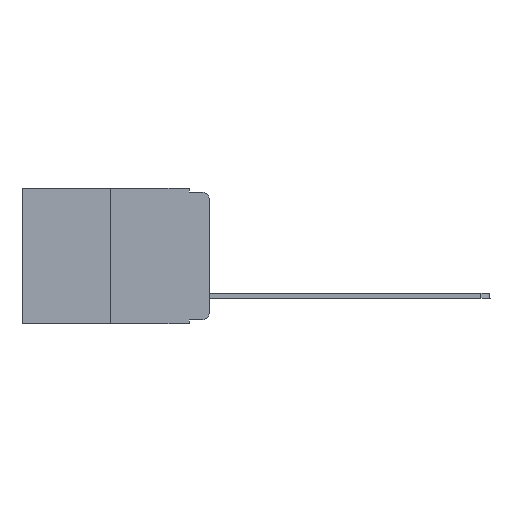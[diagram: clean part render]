
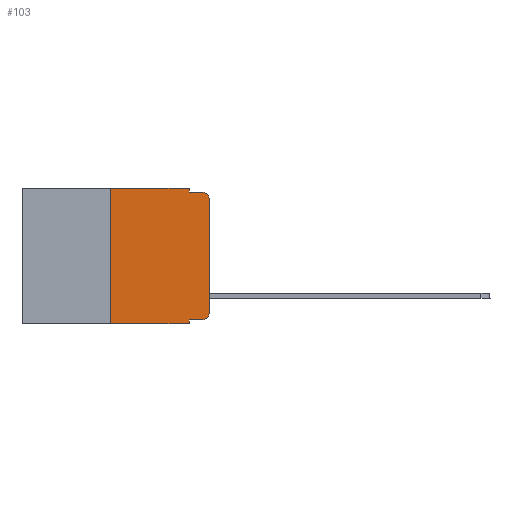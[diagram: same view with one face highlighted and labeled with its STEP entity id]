
A CAD part, left-side view. The second image highlights one B-rep face of the part: STEP entity #103.
In plain terms, the highlighted planar face has unit normal (-1, 0, 0).
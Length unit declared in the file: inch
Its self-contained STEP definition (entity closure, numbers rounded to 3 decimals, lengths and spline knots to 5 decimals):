
#103 = ADVANCED_FACE ( 'NONE', ( #1729 ), #5433, .F. ) ;
#255 = CARTESIAN_POINT ( 'NONE',  ( 0., 0.051, 0. ) ) ;
#349 = CARTESIAN_POINT ( 'NONE',  ( 0., 0.02, -0.01 ) ) ;
#372 = DIRECTION ( 'NONE',  ( 0., 0., -1. ) ) ;
#396 = EDGE_CURVE ( 'NONE', #9102, #11403, #11046, .T. ) ;
#426 = DIRECTION ( 'NONE',  ( 0., -1., 0. ) ) ;
#497 = EDGE_LOOP ( 'NONE', ( #7751, #4472, #10435, #3628, #12451, #8304, #6946, #598, #6780, #918 ) ) ;
#598 = ORIENTED_EDGE ( 'NONE', *, *, #800, .F. ) ;
#708 = VERTEX_POINT ( 'NONE', #5672 ) ;
#800 = EDGE_CURVE ( 'NONE', #7543, #8724, #7452, .T. ) ;
#918 = ORIENTED_EDGE ( 'NONE', *, *, #6258, .T. ) ;
#961 = CARTESIAN_POINT ( 'NONE',  ( 0., 0.051, 0. ) ) ;
#1445 = AXIS2_PLACEMENT_3D ( 'NONE', #3823, #12414, #6648 ) ;
#1504 = VERTEX_POINT ( 'NONE', #4629 ) ;
#1692 = VECTOR ( 'NONE', #6215, 39.37008 ) ;
#1729 = FACE_OUTER_BOUND ( 'NONE', #497, .T. ) ;
#2142 = CARTESIAN_POINT ( 'NONE',  ( 0., 0.051, 0. ) ) ;
#2344 = VECTOR ( 'NONE', #4037, 39.37008 ) ;
#2550 = CARTESIAN_POINT ( 'NONE',  ( 0., 0.02, -0.333 ) ) ;
#2570 = LINE ( 'NONE', #12297, #5564 ) ;
#2687 = EDGE_CURVE ( 'NONE', #11403, #7449, #8014, .T. ) ;
#2717 = DIRECTION ( 'NONE',  ( 1., 0., 0. ) ) ;
#2796 = VECTOR ( 'NONE', #2959, 39.37008 ) ;
#2822 = EDGE_CURVE ( 'NONE', #1504, #8724, #6805, .T. ) ;
#2959 = DIRECTION ( 'NONE',  ( 0., 0., -1. ) ) ;
#3353 = DIRECTION ( 'NONE',  ( 0., -1., 0. ) ) ;
#3569 = LINE ( 'NONE', #10056, #10960 ) ;
#3628 = ORIENTED_EDGE ( 'NONE', *, *, #396, .F. ) ;
#3698 = DIRECTION ( 'NONE',  ( 0., -1., 0. ) ) ;
#3823 = CARTESIAN_POINT ( 'NONE',  ( 0., 0.02, -0.03 ) ) ;
#4037 = DIRECTION ( 'NONE',  ( 0., 0., -1. ) ) ;
#4445 = CARTESIAN_POINT ( 'NONE',  ( 0., 0.051, -0.333 ) ) ;
#4455 = CARTESIAN_POINT ( 'NONE',  ( 0., 0.25, 0. ) ) ;
#4472 = ORIENTED_EDGE ( 'NONE', *, *, #6532, .T. ) ;
#4629 = CARTESIAN_POINT ( 'NONE',  ( 0., 0.25, -0.343 ) ) ;
#5057 = EDGE_CURVE ( 'NONE', #7543, #6416, #3569, .T. ) ;
#5117 = VERTEX_POINT ( 'NONE', #11272 ) ;
#5433 = PLANE ( 'NONE',  #8969 ) ;
#5476 = DIRECTION ( 'NONE',  ( 0., 0., -1. ) ) ;
#5564 = VECTOR ( 'NONE', #9657, 39.37008 ) ;
#5672 = CARTESIAN_POINT ( 'NONE',  ( 0., 0., -0.313 ) ) ;
#6215 = DIRECTION ( 'NONE',  ( 0., -1., 0. ) ) ;
#6258 = EDGE_CURVE ( 'NONE', #6416, #708, #7625, .T. ) ;
#6416 = VERTEX_POINT ( 'NONE', #2550 ) ;
#6532 = EDGE_CURVE ( 'NONE', #5117, #7449, #12420, .T. ) ;
#6605 = EDGE_CURVE ( 'NONE', #708, #5117, #11222, .T. ) ;
#6648 = DIRECTION ( 'NONE',  ( 0., 0., -1. ) ) ;
#6780 = ORIENTED_EDGE ( 'NONE', *, *, #5057, .T. ) ;
#6805 = LINE ( 'NONE', #10054, #1692 ) ;
#6946 = ORIENTED_EDGE ( 'NONE', *, *, #2822, .T. ) ;
#7155 = CARTESIAN_POINT ( 'NONE',  ( 0., 0.02, -0.313 ) ) ;
#7449 = VERTEX_POINT ( 'NONE', #349 ) ;
#7452 = LINE ( 'NONE', #961, #2796 ) ;
#7458 = EDGE_CURVE ( 'NONE', #8678, #9102, #12241, .T. ) ;
#7543 = VERTEX_POINT ( 'NONE', #4445 ) ;
#7612 = CARTESIAN_POINT ( 'NONE',  ( 0., 0.051, -0.01 ) ) ;
#7625 = CIRCLE ( 'NONE', #7739, 0.02 ) ;
#7739 = AXIS2_PLACEMENT_3D ( 'NONE', #7155, #11958, #372 ) ;
#7751 = ORIENTED_EDGE ( 'NONE', *, *, #6605, .T. ) ;
#8014 = LINE ( 'NONE', #12486, #9520 ) ;
#8304 = ORIENTED_EDGE ( 'NONE', *, *, #9202, .F. ) ;
#8678 = VERTEX_POINT ( 'NONE', #4455 ) ;
#8724 = VERTEX_POINT ( 'NONE', #10175 ) ;
#8781 = VECTOR ( 'NONE', #426, 39.37008 ) ;
#8969 = AXIS2_PLACEMENT_3D ( 'NONE', #9277, #2717, #5476 ) ;
#9102 = VERTEX_POINT ( 'NONE', #255 ) ;
#9202 = EDGE_CURVE ( 'NONE', #1504, #8678, #2570, .T. ) ;
#9277 = CARTESIAN_POINT ( 'NONE',  ( 0., 0.473, 0. ) ) ;
#9520 = VECTOR ( 'NONE', #3698, 39.37008 ) ;
#9657 = DIRECTION ( 'NONE',  ( 0., 0., 1. ) ) ;
#9677 = CARTESIAN_POINT ( 'NONE',  ( 0., 0., 0. ) ) ;
#10054 = CARTESIAN_POINT ( 'NONE',  ( 0., 0.473, -0.343 ) ) ;
#10056 = CARTESIAN_POINT ( 'NONE',  ( 0., 0.051, -0.333 ) ) ;
#10175 = CARTESIAN_POINT ( 'NONE',  ( 0., 0.051, -0.343 ) ) ;
#10435 = ORIENTED_EDGE ( 'NONE', *, *, #2687, .F. ) ;
#10474 = VECTOR ( 'NONE', #10777, 39.37008 ) ;
#10777 = DIRECTION ( 'NONE',  ( 0., 0., 1. ) ) ;
#10960 = VECTOR ( 'NONE', #3353, 39.37008 ) ;
#11046 = LINE ( 'NONE', #2142, #2344 ) ;
#11171 = CARTESIAN_POINT ( 'NONE',  ( 0., 0.473, 0. ) ) ;
#11222 = LINE ( 'NONE', #9677, #10474 ) ;
#11272 = CARTESIAN_POINT ( 'NONE',  ( 0., 0., -0.03 ) ) ;
#11403 = VERTEX_POINT ( 'NONE', #7612 ) ;
#11958 = DIRECTION ( 'NONE',  ( -1., 0., 0. ) ) ;
#12241 = LINE ( 'NONE', #11171, #8781 ) ;
#12297 = CARTESIAN_POINT ( 'NONE',  ( 0., 0.25, 0. ) ) ;
#12414 = DIRECTION ( 'NONE',  ( -1., 0., 0. ) ) ;
#12420 = CIRCLE ( 'NONE', #1445, 0.02 ) ;
#12451 = ORIENTED_EDGE ( 'NONE', *, *, #7458, .F. ) ;
#12486 = CARTESIAN_POINT ( 'NONE',  ( 0., 0.051, -0.01 ) ) ;
